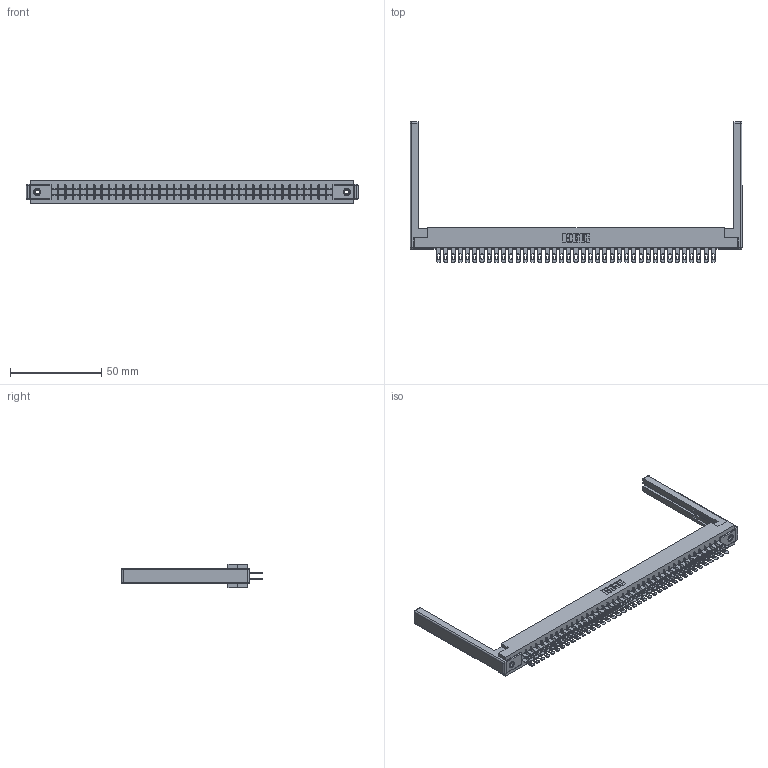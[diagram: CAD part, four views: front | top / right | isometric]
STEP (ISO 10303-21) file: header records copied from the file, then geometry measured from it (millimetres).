
FILE_DESCRIPTION (( 'STEP AP203' ), '1' );
FILE_NAME ('305-078-500-268.STEP', '2019-09-10T08:36:57', ( '' ), ( '' ), 'SwSTEP 2.0', 'SolidWorks 2016', '' );
FILE_SCHEMA (( 'CONFIG_CONTROL_DESIGN' ));
Length unit declared in the file: inch
Products named in the file (5): 305 Part_.156 Dia; 305-290-001_500; 307-220-068; 305-078-500-268; 345-250-001_345-250-001-102
Assembly tree (83 placements, depth 2):
  305-078-500-268
    305 Part_.156 Dia
    305-290-001_500  x78
    345-250-001_345-250-001-102  x2
    307-220-068  x2
Bounding box: 181.97 x 77.14 x 12.7 mm (x, y, z)
Volume: 23589.6 mm3; surface area: 29868.5 mm2
Topology: 83 solids, 83 shells, 4170 faces, 11899 edges, 7702 vertices
Faces by surface type: plane 2340, cylinder 1650, sphere 164, cone 12, torus 4
Entity records: 45373 total; most frequent: CARTESIAN_POINT 7480, ORIENTED_EDGE 7416, DIRECTION 7260, EDGE_CURVE 3708, VECTOR 2984, LINE 2984, VERTEX_POINT 2358, AXIS2_PLACEMENT_3D 2138
